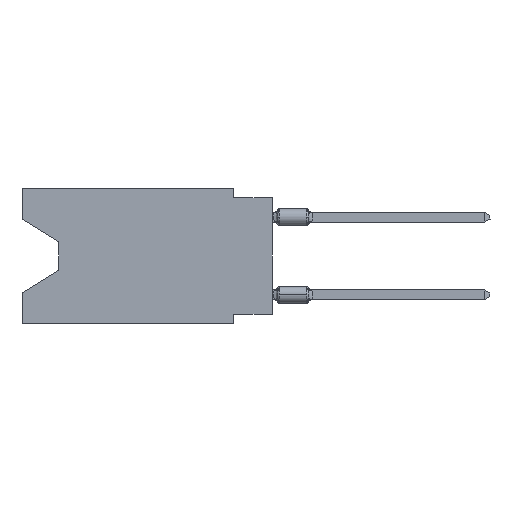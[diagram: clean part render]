
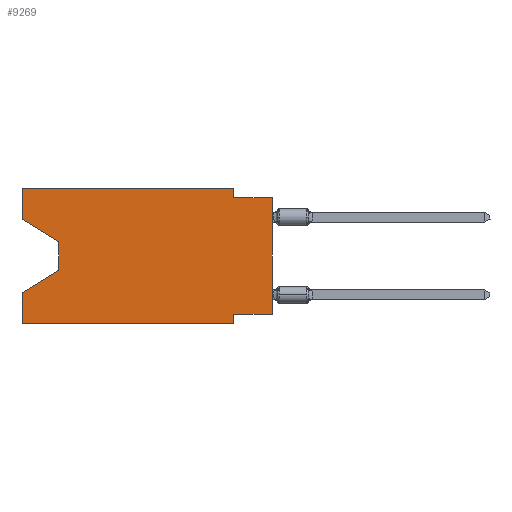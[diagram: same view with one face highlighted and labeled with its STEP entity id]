
A CAD part, left-side view. The second image highlights one B-rep face of the part: STEP entity #9269.
In plain terms, the highlighted planar face has unit normal (-1, 0, 0).
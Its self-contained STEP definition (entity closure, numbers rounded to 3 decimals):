
#201 = ORIENTED_EDGE ( 'NONE', *, *, #7190, .T. ) ;
#687 = CARTESIAN_POINT ( 'NONE',  ( 0., 13.97, -5.385 ) ) ;
#1341 = ORIENTED_EDGE ( 'NONE', *, *, #28291, .T. ) ;
#1411 = DIRECTION ( 'NONE',  ( 0., 0.855, -0.519 ) ) ;
#1589 = VECTOR ( 'NONE', #13795, 1000. ) ;
#1665 = CARTESIAN_POINT ( 'NONE',  ( 0., 16.383, 0. ) ) ;
#2170 = EDGE_CURVE ( 'NONE', #28678, #19084, #3669, .T. ) ;
#2241 = DIRECTION ( 'NONE',  ( 0., 0., -1. ) ) ;
#2432 = CARTESIAN_POINT ( 'NONE',  ( 0., 2.54, -8.255 ) ) ;
#3669 = LINE ( 'NONE', #14499, #7974 ) ;
#3910 = VECTOR ( 'NONE', #16306, 1000. ) ;
#4805 = DIRECTION ( 'NONE',  ( 0., 0., 1. ) ) ;
#5019 = EDGE_CURVE ( 'NONE', #33153, #9888, #26005, .T. ) ;
#5867 = LINE ( 'NONE', #11188, #24116 ) ;
#5914 = CARTESIAN_POINT ( 'NONE',  ( 0., 13.97, -3.505 ) ) ;
#6978 = DIRECTION ( 'NONE',  ( 0., -1., 0. ) ) ;
#7072 = CARTESIAN_POINT ( 'NONE',  ( 0., 16.383, -2.038 ) ) ;
#7190 = EDGE_CURVE ( 'NONE', #15556, #20070, #20951, .T. ) ;
#7533 = CARTESIAN_POINT ( 'NONE',  ( 0., 2.54, -8.89 ) ) ;
#7974 = VECTOR ( 'NONE', #25346, 1000. ) ;
#8095 = CARTESIAN_POINT ( 'NONE',  ( 0., 0., -0.635 ) ) ;
#8712 = EDGE_CURVE ( 'NONE', #28678, #25796, #26444, .T. ) ;
#9269 = ADVANCED_FACE ( 'NONE', ( #17320 ), #28337, .F. ) ;
#9888 = VERTEX_POINT ( 'NONE', #28810 ) ;
#9906 = EDGE_LOOP ( 'NONE', ( #201, #34126, #14371, #13026, #17182, #17383, #13775, #1341, #11734, #16654, #21060, #30942 ) ) ;
#9930 = CARTESIAN_POINT ( 'NONE',  ( 0., 13.97, -5.385 ) ) ;
#10278 = DIRECTION ( 'NONE',  ( 0., 0., 1. ) ) ;
#10578 = CARTESIAN_POINT ( 'NONE',  ( 0., 16.383, -8.89 ) ) ;
#11149 = DIRECTION ( 'NONE',  ( 0., 0., 1. ) ) ;
#11188 = CARTESIAN_POINT ( 'NONE',  ( 0., 2.54, 0. ) ) ;
#11734 = ORIENTED_EDGE ( 'NONE', *, *, #34651, .F. ) ;
#13026 = ORIENTED_EDGE ( 'NONE', *, *, #8712, .F. ) ;
#13775 = ORIENTED_EDGE ( 'NONE', *, *, #22802, .F. ) ;
#13795 = DIRECTION ( 'NONE',  ( 0., -1., 0. ) ) ;
#14371 = ORIENTED_EDGE ( 'NONE', *, *, #18165, .T. ) ;
#14499 = CARTESIAN_POINT ( 'NONE',  ( 0., 16.383, -8.89 ) ) ;
#15251 = VERTEX_POINT ( 'NONE', #2432 ) ;
#15356 = CARTESIAN_POINT ( 'NONE',  ( 0., 0., -0.635 ) ) ;
#15556 = VERTEX_POINT ( 'NONE', #31552 ) ;
#16306 = DIRECTION ( 'NONE',  ( 0., 1., 0. ) ) ;
#16595 = CARTESIAN_POINT ( 'NONE',  ( 0., 16.383, -6.852 ) ) ;
#16654 = ORIENTED_EDGE ( 'NONE', *, *, #16776, .F. ) ;
#16761 = DIRECTION ( 'NONE',  ( 0., 0., -1. ) ) ;
#16776 = EDGE_CURVE ( 'NONE', #9888, #19008, #5867, .T. ) ;
#17032 = CARTESIAN_POINT ( 'NONE',  ( 0., 16.383, 0. ) ) ;
#17182 = ORIENTED_EDGE ( 'NONE', *, *, #2170, .T. ) ;
#17218 = VECTOR ( 'NONE', #6978, 1000. ) ;
#17320 = FACE_OUTER_BOUND ( 'NONE', #9906, .T. ) ;
#17383 = ORIENTED_EDGE ( 'NONE', *, *, #25363, .F. ) ;
#17519 = VECTOR ( 'NONE', #16761, 1000. ) ;
#17931 = DIRECTION ( 'NONE',  ( 0., -0.855, -0.519 ) ) ;
#18165 = EDGE_CURVE ( 'NONE', #19632, #25796, #28438, .T. ) ;
#18446 = CARTESIAN_POINT ( 'NONE',  ( 0., 16.383, 0. ) ) ;
#18490 = VECTOR ( 'NONE', #10278, 1000. ) ;
#19008 = VERTEX_POINT ( 'NONE', #25318 ) ;
#19084 = VERTEX_POINT ( 'NONE', #7533 ) ;
#19632 = VERTEX_POINT ( 'NONE', #687 ) ;
#20070 = VERTEX_POINT ( 'NONE', #32231 ) ;
#20370 = VERTEX_POINT ( 'NONE', #15356 ) ;
#20639 = LINE ( 'NONE', #29162, #23677 ) ;
#20951 = LINE ( 'NONE', #7072, #32934 ) ;
#21060 = ORIENTED_EDGE ( 'NONE', *, *, #5019, .F. ) ;
#21982 = CARTESIAN_POINT ( 'NONE',  ( 0., 0., -8.255 ) ) ;
#22223 = DIRECTION ( 'NONE',  ( 0., 0., -1. ) ) ;
#22467 = DIRECTION ( 'NONE',  ( 1., 0., 0. ) ) ;
#22802 = EDGE_CURVE ( 'NONE', #26352, #15251, #29645, .T. ) ;
#23654 = CARTESIAN_POINT ( 'NONE',  ( 0., 0., 0. ) ) ;
#23677 = VECTOR ( 'NONE', #4805, 1000. ) ;
#24116 = VECTOR ( 'NONE', #22223, 1000. ) ;
#24276 = LINE ( 'NONE', #8095, #1589 ) ;
#24361 = VECTOR ( 'NONE', #11149, 1000. ) ;
#24670 = LINE ( 'NONE', #23654, #24361 ) ;
#25149 = CARTESIAN_POINT ( 'NONE',  ( 0., 16.383, 0. ) ) ;
#25318 = CARTESIAN_POINT ( 'NONE',  ( 0., 2.54, -0.635 ) ) ;
#25346 = DIRECTION ( 'NONE',  ( 0., -1., 0. ) ) ;
#25363 = EDGE_CURVE ( 'NONE', #15251, #19084, #26590, .T. ) ;
#25796 = VERTEX_POINT ( 'NONE', #16595 ) ;
#25983 = VECTOR ( 'NONE', #2241, 1000. ) ;
#26005 = LINE ( 'NONE', #1665, #17218 ) ;
#26352 = VERTEX_POINT ( 'NONE', #34435 ) ;
#26444 = LINE ( 'NONE', #18446, #18490 ) ;
#26590 = LINE ( 'NONE', #35136, #25983 ) ;
#27123 = EDGE_CURVE ( 'NONE', #20070, #19632, #30279, .T. ) ;
#28145 = DIRECTION ( 'NONE',  ( 0., 0., -1. ) ) ;
#28291 = EDGE_CURVE ( 'NONE', #26352, #20370, #24670, .T. ) ;
#28337 = PLANE ( 'NONE',  #33303 ) ;
#28438 = LINE ( 'NONE', #9930, #29000 ) ;
#28678 = VERTEX_POINT ( 'NONE', #10578 ) ;
#28810 = CARTESIAN_POINT ( 'NONE',  ( 0., 2.54, 0. ) ) ;
#29000 = VECTOR ( 'NONE', #1411, 1000. ) ;
#29162 = CARTESIAN_POINT ( 'NONE',  ( 0., 16.383, 0. ) ) ;
#29645 = LINE ( 'NONE', #21982, #3910 ) ;
#30279 = LINE ( 'NONE', #5914, #17519 ) ;
#30942 = ORIENTED_EDGE ( 'NONE', *, *, #33610, .F. ) ;
#31552 = CARTESIAN_POINT ( 'NONE',  ( 0., 16.383, -2.038 ) ) ;
#32231 = CARTESIAN_POINT ( 'NONE',  ( 0., 13.97, -3.505 ) ) ;
#32934 = VECTOR ( 'NONE', #17931, 1000. ) ;
#33153 = VERTEX_POINT ( 'NONE', #17032 ) ;
#33303 = AXIS2_PLACEMENT_3D ( 'NONE', #25149, #22467, #28145 ) ;
#33610 = EDGE_CURVE ( 'NONE', #15556, #33153, #20639, .T. ) ;
#34126 = ORIENTED_EDGE ( 'NONE', *, *, #27123, .T. ) ;
#34435 = CARTESIAN_POINT ( 'NONE',  ( 0., 0., -8.255 ) ) ;
#34651 = EDGE_CURVE ( 'NONE', #19008, #20370, #24276, .T. ) ;
#35136 = CARTESIAN_POINT ( 'NONE',  ( 0., 2.54, -8.89 ) ) ;
